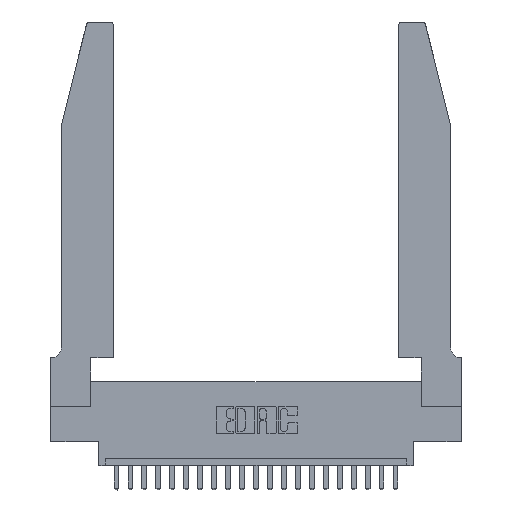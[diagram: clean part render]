
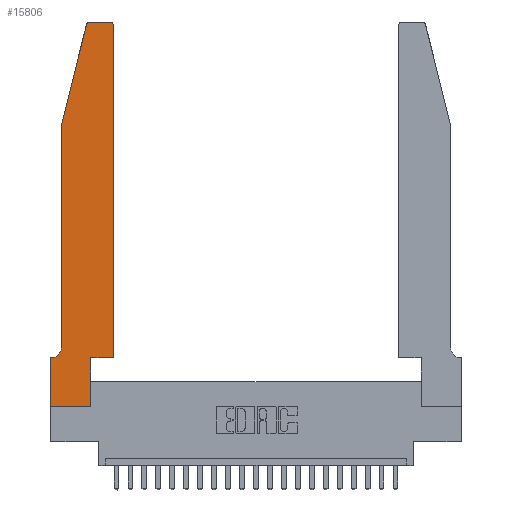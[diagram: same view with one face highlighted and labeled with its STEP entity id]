
A CAD part, top view. The second image highlights one B-rep face of the part: STEP entity #15806.
In plain terms, the highlighted planar face has unit normal (0, 0, 1).
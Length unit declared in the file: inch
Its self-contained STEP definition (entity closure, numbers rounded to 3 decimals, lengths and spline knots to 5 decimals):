
#75 = CARTESIAN_POINT ( 'NONE',  ( 0.0755, 0.35, 0.37 ) ) ;
#81 = ORIENTED_EDGE ( 'NONE', *, *, #1915, .T. ) ;
#575 = EDGE_CURVE ( 'NONE', #4191, #2423, #12350, .T. ) ;
#646 = EDGE_CURVE ( 'NONE', #2423, #12652, #6926, .T. ) ;
#1003 = DIRECTION ( 'NONE',  ( 0., -1., 0. ) ) ;
#1059 = CARTESIAN_POINT ( 'NONE',  ( 0.0755, 2., 0.37 ) ) ;
#1375 = VECTOR ( 'NONE', #14936, 39.37008 ) ;
#1399 = VERTEX_POINT ( 'NONE', #4485 ) ;
#1915 = EDGE_CURVE ( 'NONE', #16703, #10123, #8281, .T. ) ;
#2176 = DIRECTION ( 'NONE',  ( 0., 1., 0. ) ) ;
#2423 = VERTEX_POINT ( 'NONE', #4257 ) ;
#2462 = CIRCLE ( 'NONE', #19828, 0.03 ) ;
#2996 = EDGE_LOOP ( 'NONE', ( #4447, #81, #6729, #7084, #23431, #6795, #18466, #10503, #10429, #6355, #4362, #13634 ) ) ;
#3175 = VECTOR ( 'NONE', #14549, 39.37008 ) ;
#3725 = DIRECTION ( 'NONE',  ( -1., 0., 0. ) ) ;
#4191 = VERTEX_POINT ( 'NONE', #22575 ) ;
#4216 = VECTOR ( 'NONE', #6033, 39.37008 ) ;
#4257 = CARTESIAN_POINT ( 'NONE',  ( 0., 0.35, 0.37 ) ) ;
#4362 = ORIENTED_EDGE ( 'NONE', *, *, #17597, .T. ) ;
#4371 = DIRECTION ( 'NONE',  ( 0., 0., 1. ) ) ;
#4447 = ORIENTED_EDGE ( 'NONE', *, *, #21479, .T. ) ;
#4485 = CARTESIAN_POINT ( 'NONE',  ( 0.2865, 0., 0.37 ) ) ;
#4812 = AXIS2_PLACEMENT_3D ( 'NONE', #5292, #19889, #9042 ) ;
#4989 = CARTESIAN_POINT ( 'NONE',  ( 0.2865, 0.35, 0.37 ) ) ;
#5010 = CARTESIAN_POINT ( 'NONE',  ( 0.0755, 0.42, 0.37 ) ) ;
#5093 = LINE ( 'NONE', #10372, #15375 ) ;
#5292 = CARTESIAN_POINT ( 'NONE',  ( 0.0055, 0.42, 0.37 ) ) ;
#5582 = VERTEX_POINT ( 'NONE', #13678 ) ;
#5655 = DIRECTION ( 'NONE',  ( 0., 0., 1. ) ) ;
#6033 = DIRECTION ( 'NONE',  ( -1., 0., 0. ) ) ;
#6355 = ORIENTED_EDGE ( 'NONE', *, *, #8429, .T. ) ;
#6619 = CARTESIAN_POINT ( 'NONE',  ( 0.25487, 2.72718, 0.37 ) ) ;
#6729 = ORIENTED_EDGE ( 'NONE', *, *, #16829, .T. ) ;
#6795 = ORIENTED_EDGE ( 'NONE', *, *, #575, .T. ) ;
#6926 = LINE ( 'NONE', #12699, #3175 ) ;
#7084 = ORIENTED_EDGE ( 'NONE', *, *, #22559, .T. ) ;
#7477 = DIRECTION ( 'NONE',  ( 1., 0., 0. ) ) ;
#8213 = VERTEX_POINT ( 'NONE', #13812 ) ;
#8250 = LINE ( 'NONE', #11966, #16816 ) ;
#8281 = CIRCLE ( 'NONE', #9142, 0.03 ) ;
#8429 = EDGE_CURVE ( 'NONE', #18367, #20131, #16951, .T. ) ;
#8486 = LINE ( 'NONE', #11322, #13912 ) ;
#8794 = CARTESIAN_POINT ( 'NONE',  ( 0., 0., 0.37 ) ) ;
#9031 = EDGE_CURVE ( 'NONE', #21111, #4191, #13079, .T. ) ;
#9042 = DIRECTION ( 'NONE',  ( -1., 0., 0. ) ) ;
#9142 = AXIS2_PLACEMENT_3D ( 'NONE', #9741, #4371, #22481 ) ;
#9667 = DIRECTION ( 'NONE',  ( 1., 0., 0. ) ) ;
#9741 = CARTESIAN_POINT ( 'NONE',  ( 0.284, 2.72, 0.37 ) ) ;
#9742 = PLANE ( 'NONE',  #20033 ) ;
#10123 = VERTEX_POINT ( 'NONE', #6619 ) ;
#10260 = LINE ( 'NONE', #12869, #1375 ) ;
#10372 = CARTESIAN_POINT ( 'NONE',  ( 0.0755, 2., 0.37 ) ) ;
#10429 = ORIENTED_EDGE ( 'NONE', *, *, #18147, .T. ) ;
#10503 = ORIENTED_EDGE ( 'NONE', *, *, #14183, .T. ) ;
#11322 = CARTESIAN_POINT ( 'NONE',  ( 0.4505, 0.35, 0.37 ) ) ;
#11536 = CARTESIAN_POINT ( 'NONE',  ( 0.2605, 2.75, 0.37 ) ) ;
#11775 = VECTOR ( 'NONE', #3725, 39.37008 ) ;
#11966 = CARTESIAN_POINT ( 'NONE',  ( 0., 0., 0.37 ) ) ;
#12350 = LINE ( 'NONE', #75, #11775 ) ;
#12479 = LINE ( 'NONE', #4989, #13059 ) ;
#12504 = CARTESIAN_POINT ( 'NONE',  ( 0.4505, 0.35, 0.37 ) ) ;
#12652 = VERTEX_POINT ( 'NONE', #8794 ) ;
#12699 = CARTESIAN_POINT ( 'NONE',  ( 0., 0., 0.37 ) ) ;
#12869 = CARTESIAN_POINT ( 'NONE',  ( 0.0755, 2., 0.37 ) ) ;
#12972 = CARTESIAN_POINT ( 'NONE',  ( 0.2865, 0.35, 0.37 ) ) ;
#13059 = VECTOR ( 'NONE', #15851, 39.37008 ) ;
#13079 = CIRCLE ( 'NONE', #4812, 0.07 ) ;
#13634 = ORIENTED_EDGE ( 'NONE', *, *, #22827, .T. ) ;
#13678 = CARTESIAN_POINT ( 'NONE',  ( 0.4205, 2.75, 0.37 ) ) ;
#13812 = CARTESIAN_POINT ( 'NONE',  ( 0.4505, 2.72, 0.37 ) ) ;
#13912 = VECTOR ( 'NONE', #2176, 39.37008 ) ;
#14183 = EDGE_CURVE ( 'NONE', #12652, #1399, #8250, .T. ) ;
#14549 = DIRECTION ( 'NONE',  ( 0., -1., 0. ) ) ;
#14817 = LINE ( 'NONE', #11536, #4216 ) ;
#14936 = DIRECTION ( 'NONE',  ( -0.239, -0.971, 0. ) ) ;
#14950 = DIRECTION ( 'NONE',  ( 0., 0., 1. ) ) ;
#15304 = CARTESIAN_POINT ( 'NONE',  ( 0.4505, 0.35, 0.37 ) ) ;
#15375 = VECTOR ( 'NONE', #1003, 39.37008 ) ;
#15806 = ADVANCED_FACE ( 'NONE', ( #16308 ), #9742, .T. ) ;
#15851 = DIRECTION ( 'NONE',  ( 0., 1., 0. ) ) ;
#16175 = DIRECTION ( 'NONE',  ( 1., 0., 0. ) ) ;
#16308 = FACE_OUTER_BOUND ( 'NONE', #2996, .T. ) ;
#16508 = CARTESIAN_POINT ( 'NONE',  ( 0.4205, 2.72, 0.37 ) ) ;
#16703 = VERTEX_POINT ( 'NONE', #18361 ) ;
#16816 = VECTOR ( 'NONE', #22734, 39.37008 ) ;
#16829 = EDGE_CURVE ( 'NONE', #10123, #18132, #10260, .T. ) ;
#16951 = LINE ( 'NONE', #12504, #19811 ) ;
#17597 = EDGE_CURVE ( 'NONE', #20131, #8213, #8486, .T. ) ;
#18132 = VERTEX_POINT ( 'NONE', #1059 ) ;
#18147 = EDGE_CURVE ( 'NONE', #1399, #18367, #12479, .T. ) ;
#18361 = CARTESIAN_POINT ( 'NONE',  ( 0.284, 2.75, 0.37 ) ) ;
#18367 = VERTEX_POINT ( 'NONE', #12972 ) ;
#18466 = ORIENTED_EDGE ( 'NONE', *, *, #646, .T. ) ;
#19811 = VECTOR ( 'NONE', #16175, 39.37008 ) ;
#19828 = AXIS2_PLACEMENT_3D ( 'NONE', #16508, #5655, #7477 ) ;
#19889 = DIRECTION ( 'NONE',  ( 0., 0., -1. ) ) ;
#20033 = AXIS2_PLACEMENT_3D ( 'NONE', #22482, #14950, #9667 ) ;
#20131 = VERTEX_POINT ( 'NONE', #15304 ) ;
#21111 = VERTEX_POINT ( 'NONE', #5010 ) ;
#21479 = EDGE_CURVE ( 'NONE', #5582, #16703, #14817, .T. ) ;
#22481 = DIRECTION ( 'NONE',  ( 1., 0., 0. ) ) ;
#22482 = CARTESIAN_POINT ( 'NONE',  ( 0., 0.35, 0.37 ) ) ;
#22559 = EDGE_CURVE ( 'NONE', #18132, #21111, #5093, .T. ) ;
#22575 = CARTESIAN_POINT ( 'NONE',  ( 0.0055, 0.35, 0.37 ) ) ;
#22734 = DIRECTION ( 'NONE',  ( 1., 0., 0. ) ) ;
#22827 = EDGE_CURVE ( 'NONE', #8213, #5582, #2462, .T. ) ;
#23431 = ORIENTED_EDGE ( 'NONE', *, *, #9031, .T. ) ;
